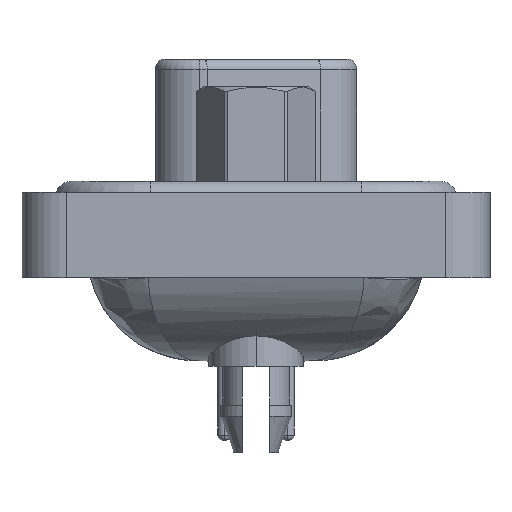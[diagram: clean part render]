
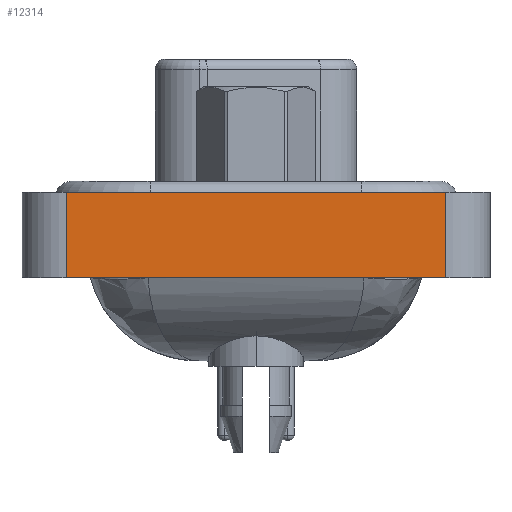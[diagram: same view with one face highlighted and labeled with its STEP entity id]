
A CAD part, left-side view. The second image highlights one B-rep face of the part: STEP entity #12314.
In plain terms, the highlighted planar face has unit normal (-1, 0, 0).
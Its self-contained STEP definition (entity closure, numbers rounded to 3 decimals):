
#324 = ORIENTED_EDGE ( 'NONE', *, *, #6822, .F. ) ;
#748 = EDGE_CURVE ( 'NONE', #27154, #8489, #1185, .T. ) ;
#965 = CARTESIAN_POINT ( 'NONE',  ( -7.225, -8.55, 0.5 ) ) ;
#1185 = LINE ( 'NONE', #23259, #12185 ) ;
#2410 = DIRECTION ( 'NONE',  ( 0., 0., 1. ) ) ;
#3084 = DIRECTION ( 'NONE',  ( 0., -1., 0. ) ) ;
#3229 = DIRECTION ( 'NONE',  ( 0., 0., 1. ) ) ;
#5951 = EDGE_CURVE ( 'NONE', #8489, #9506, #23198, .T. ) ;
#6692 = PLANE ( 'NONE',  #27083 ) ;
#6822 = EDGE_CURVE ( 'NONE', #27154, #21939, #17929, .T. ) ;
#8103 = EDGE_CURVE ( 'NONE', #21939, #9506, #20723, .T. ) ;
#8489 = VERTEX_POINT ( 'NONE', #16220 ) ;
#9506 = VERTEX_POINT ( 'NONE', #14633 ) ;
#10784 = ORIENTED_EDGE ( 'NONE', *, *, #748, .T. ) ;
#11455 = VECTOR ( 'NONE', #18572, 1000. ) ;
#12076 = CARTESIAN_POINT ( 'NONE',  ( -7.225, -8.55, -3.35 ) ) ;
#12185 = VECTOR ( 'NONE', #3084, 1000. ) ;
#12314 = ADVANCED_FACE ( 'NONE', ( #24773 ), #6692, .T. ) ;
#14249 = VECTOR ( 'NONE', #3229, 1000. ) ;
#14633 = CARTESIAN_POINT ( 'NONE',  ( -7.225, -8.55, 0.5 ) ) ;
#15807 = CARTESIAN_POINT ( 'NONE',  ( -7.225, -8.55, -3.35 ) ) ;
#16220 = CARTESIAN_POINT ( 'NONE',  ( -7.225, -8.55, -3.35 ) ) ;
#17535 = DIRECTION ( 'NONE',  ( -1., 0., 0. ) ) ;
#17929 = LINE ( 'NONE', #26769, #14249 ) ;
#18572 = DIRECTION ( 'NONE',  ( 0., 0., 1. ) ) ;
#18664 = ORIENTED_EDGE ( 'NONE', *, *, #5951, .T. ) ;
#18926 = CARTESIAN_POINT ( 'NONE',  ( -7.225, 8.55, 0.5 ) ) ;
#19398 = EDGE_LOOP ( 'NONE', ( #18664, #24801, #324, #10784 ) ) ;
#20414 = VECTOR ( 'NONE', #20573, 1000. ) ;
#20573 = DIRECTION ( 'NONE',  ( 0., -1., 0. ) ) ;
#20723 = LINE ( 'NONE', #965, #20414 ) ;
#21939 = VERTEX_POINT ( 'NONE', #18926 ) ;
#23198 = LINE ( 'NONE', #12076, #11455 ) ;
#23259 = CARTESIAN_POINT ( 'NONE',  ( -7.225, -8.55, -3.35 ) ) ;
#23313 = CARTESIAN_POINT ( 'NONE',  ( -7.225, 8.55, -3.35 ) ) ;
#24773 = FACE_OUTER_BOUND ( 'NONE', #19398, .T. ) ;
#24801 = ORIENTED_EDGE ( 'NONE', *, *, #8103, .F. ) ;
#26769 = CARTESIAN_POINT ( 'NONE',  ( -7.225, 8.55, -3.35 ) ) ;
#27083 = AXIS2_PLACEMENT_3D ( 'NONE', #15807, #17535, #2410 ) ;
#27154 = VERTEX_POINT ( 'NONE', #23313 ) ;
